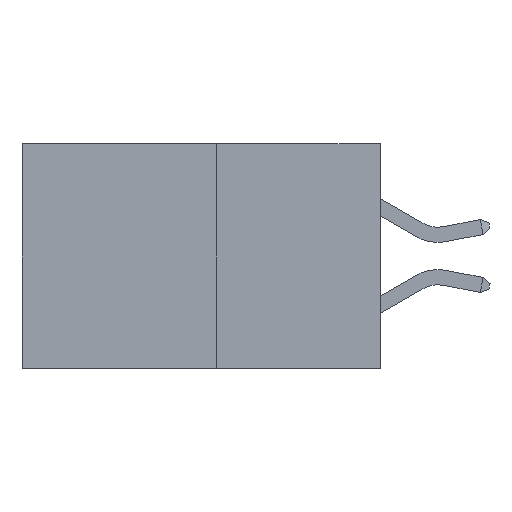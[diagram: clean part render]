
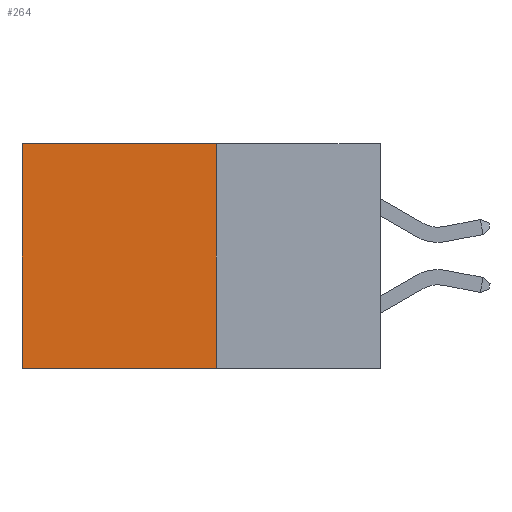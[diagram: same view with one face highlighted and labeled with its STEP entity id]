
A CAD part, left-side view. The second image highlights one B-rep face of the part: STEP entity #264.
In plain terms, the highlighted planar face has unit normal (-1, 0, 0).
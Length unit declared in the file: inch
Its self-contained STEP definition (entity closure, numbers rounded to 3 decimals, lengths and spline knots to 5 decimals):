
#264 = ADVANCED_FACE ( 'NONE', ( #4482 ), #13778, .F. ) ;
#468 = CARTESIAN_POINT ( 'NONE',  ( 0.277, 0.27, 0. ) ) ;
#538 = DIRECTION ( 'NONE',  ( 0., 1., 0. ) ) ;
#1115 = ORIENTED_EDGE ( 'NONE', *, *, #9534, .T. ) ;
#1206 = EDGE_CURVE ( 'NONE', #13686, #6501, #15740, .T. ) ;
#1948 = ORIENTED_EDGE ( 'NONE', *, *, #1206, .T. ) ;
#2118 = EDGE_LOOP ( 'NONE', ( #1948, #17636, #3446, #1115 ) ) ;
#3446 = ORIENTED_EDGE ( 'NONE', *, *, #5114, .F. ) ;
#3502 = CARTESIAN_POINT ( 'NONE',  ( 0.277, 0.27, -0.37 ) ) ;
#3887 = VECTOR ( 'NONE', #20126, 39.37008 ) ;
#3912 = DIRECTION ( 'NONE',  ( 0., 0., -1. ) ) ;
#4110 = EDGE_CURVE ( 'NONE', #7636, #6501, #13164, .T. ) ;
#4217 = CARTESIAN_POINT ( 'NONE',  ( 0.277, 0.27, -0.37 ) ) ;
#4482 = FACE_OUTER_BOUND ( 'NONE', #2118, .T. ) ;
#5114 = EDGE_CURVE ( 'NONE', #19658, #7636, #10857, .T. ) ;
#5475 = CARTESIAN_POINT ( 'NONE',  ( 0.277, 0.59, 0. ) ) ;
#6501 = VERTEX_POINT ( 'NONE', #9888 ) ;
#7127 = VECTOR ( 'NONE', #19120, 39.37008 ) ;
#7521 = VECTOR ( 'NONE', #538, 39.37008 ) ;
#7636 = VERTEX_POINT ( 'NONE', #18178 ) ;
#8944 = AXIS2_PLACEMENT_3D ( 'NONE', #10790, #14754, #11078 ) ;
#9534 = EDGE_CURVE ( 'NONE', #19658, #13686, #19808, .T. ) ;
#9888 = CARTESIAN_POINT ( 'NONE',  ( 0.277, 0.59, -0.37 ) ) ;
#10790 = CARTESIAN_POINT ( 'NONE',  ( 0.277, 0.27, -0.37 ) ) ;
#10857 = LINE ( 'NONE', #4217, #14631 ) ;
#11078 = DIRECTION ( 'NONE',  ( 0., 0., -1. ) ) ;
#12783 = CARTESIAN_POINT ( 'NONE',  ( 0.277, 0.59, -0.37 ) ) ;
#13164 = LINE ( 'NONE', #3502, #3887 ) ;
#13686 = VERTEX_POINT ( 'NONE', #5475 ) ;
#13778 = PLANE ( 'NONE',  #8944 ) ;
#14631 = VECTOR ( 'NONE', #3912, 39.37008 ) ;
#14754 = DIRECTION ( 'NONE',  ( 1., 0., 0. ) ) ;
#15740 = LINE ( 'NONE', #12783, #7127 ) ;
#17636 = ORIENTED_EDGE ( 'NONE', *, *, #4110, .F. ) ;
#18178 = CARTESIAN_POINT ( 'NONE',  ( 0.277, 0.27, -0.37 ) ) ;
#19120 = DIRECTION ( 'NONE',  ( 0., 0., -1. ) ) ;
#19658 = VERTEX_POINT ( 'NONE', #20633 ) ;
#19808 = LINE ( 'NONE', #468, #7521 ) ;
#20126 = DIRECTION ( 'NONE',  ( 0., 1., 0. ) ) ;
#20633 = CARTESIAN_POINT ( 'NONE',  ( 0.277, 0.27, 0. ) ) ;
